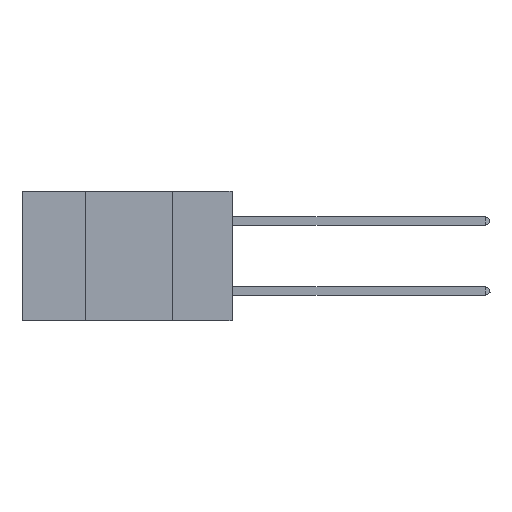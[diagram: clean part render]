
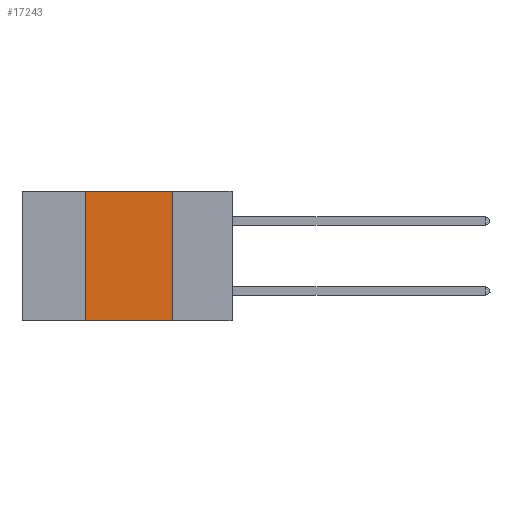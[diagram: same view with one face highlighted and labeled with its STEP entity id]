
A CAD part, left-side view. The second image highlights one B-rep face of the part: STEP entity #17243.
In plain terms, the highlighted planar face has unit normal (-1, 0, 0).
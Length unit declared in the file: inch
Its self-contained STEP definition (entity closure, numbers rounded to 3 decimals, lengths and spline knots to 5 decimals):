
#74 = VERTEX_POINT ( 'NONE', #20049 ) ;
#110 = LINE ( 'NONE', #12711, #6478 ) ;
#128 = VERTEX_POINT ( 'NONE', #18597 ) ;
#410 = DIRECTION ( 'NONE',  ( 0., 0., -1. ) ) ;
#1221 = ORIENTED_EDGE ( 'NONE', *, *, #24121, .T. ) ;
#1445 = VECTOR ( 'NONE', #20189, 39.37008 ) ;
#2268 = CARTESIAN_POINT ( 'NONE',  ( 0., 0.6, -0.37 ) ) ;
#2855 = DIRECTION ( 'NONE',  ( 1., 0., 0. ) ) ;
#3641 = ORIENTED_EDGE ( 'NONE', *, *, #20543, .F. ) ;
#4816 = VERTEX_POINT ( 'NONE', #22117 ) ;
#5299 = LINE ( 'NONE', #2268, #1445 ) ;
#5680 = DIRECTION ( 'NONE',  ( 0., 0., 1. ) ) ;
#6478 = VECTOR ( 'NONE', #8563, 39.37008 ) ;
#8563 = DIRECTION ( 'NONE',  ( 0., 0., -1. ) ) ;
#8756 = EDGE_CURVE ( 'NONE', #128, #74, #24903, .T. ) ;
#9630 = AXIS2_PLACEMENT_3D ( 'NONE', #10888, #2855, #410 ) ;
#10888 = CARTESIAN_POINT ( 'NONE',  ( 0., 0.6, 0. ) ) ;
#11270 = CARTESIAN_POINT ( 'NONE',  ( 0., 0.6, 0. ) ) ;
#12538 = EDGE_LOOP ( 'NONE', ( #3641, #20794, #14109, #1221 ) ) ;
#12711 = CARTESIAN_POINT ( 'NONE',  ( 0., 0.17, 0. ) ) ;
#13270 = VERTEX_POINT ( 'NONE', #17678 ) ;
#14109 = ORIENTED_EDGE ( 'NONE', *, *, #8756, .F. ) ;
#14819 = PLANE ( 'NONE',  #9630 ) ;
#15373 = DIRECTION ( 'NONE',  ( 0., -1., 0. ) ) ;
#15908 = LINE ( 'NONE', #11270, #19394 ) ;
#16196 = VECTOR ( 'NONE', #5680, 39.37008 ) ;
#17243 = ADVANCED_FACE ( 'NONE', ( #22975 ), #14819, .F. ) ;
#17678 = CARTESIAN_POINT ( 'NONE',  ( 0., 0.17, 0. ) ) ;
#18597 = CARTESIAN_POINT ( 'NONE',  ( 0., 0.42, -0.37 ) ) ;
#19394 = VECTOR ( 'NONE', #15373, 39.37008 ) ;
#20049 = CARTESIAN_POINT ( 'NONE',  ( 0., 0.42, 0. ) ) ;
#20189 = DIRECTION ( 'NONE',  ( 0., -1., 0. ) ) ;
#20543 = EDGE_CURVE ( 'NONE', #13270, #4816, #110, .T. ) ;
#20794 = ORIENTED_EDGE ( 'NONE', *, *, #25355, .F. ) ;
#22117 = CARTESIAN_POINT ( 'NONE',  ( 0., 0.17, -0.37 ) ) ;
#22975 = FACE_OUTER_BOUND ( 'NONE', #12538, .T. ) ;
#24121 = EDGE_CURVE ( 'NONE', #128, #4816, #5299, .T. ) ;
#24903 = LINE ( 'NONE', #25451, #16196 ) ;
#25355 = EDGE_CURVE ( 'NONE', #74, #13270, #15908, .T. ) ;
#25451 = CARTESIAN_POINT ( 'NONE',  ( 0., 0.42, 0. ) ) ;
